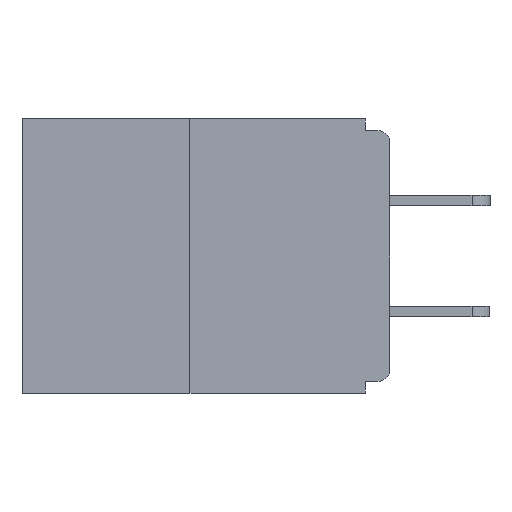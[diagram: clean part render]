
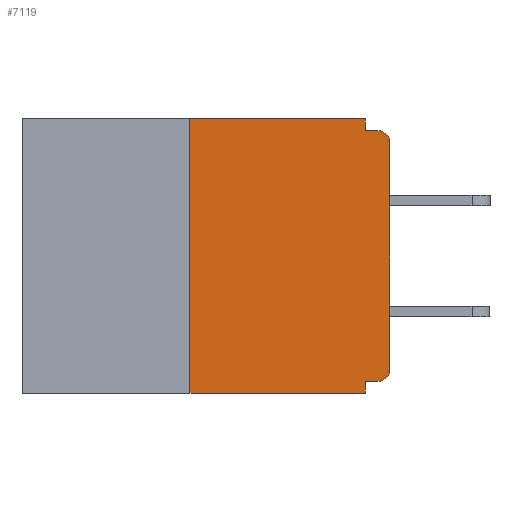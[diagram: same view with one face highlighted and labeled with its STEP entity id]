
A CAD part, left-side view. The second image highlights one B-rep face of the part: STEP entity #7119.
In plain terms, the highlighted planar face has unit normal (-1, 0, 0).
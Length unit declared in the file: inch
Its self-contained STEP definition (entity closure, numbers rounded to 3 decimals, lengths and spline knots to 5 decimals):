
#192 = DIRECTION ( 'NONE',  ( 0., 0., -1. ) ) ;
#366 = VECTOR ( 'NONE', #7528, 39.37008 ) ;
#459 = DIRECTION ( 'NONE',  ( 0., -1., 0. ) ) ;
#569 = LINE ( 'NONE', #3415, #7315 ) ;
#801 = DIRECTION ( 'NONE',  ( 0., 1., 0. ) ) ;
#1055 = LINE ( 'NONE', #1963, #10873 ) ;
#1112 = ORIENTED_EDGE ( 'NONE', *, *, #2928, .F. ) ;
#1185 = DIRECTION ( 'NONE',  ( 1., 0., 0. ) ) ;
#1282 = VERTEX_POINT ( 'NONE', #8384 ) ;
#1338 = CARTESIAN_POINT ( 'NONE',  ( 0., 0., -0.015 ) ) ;
#1354 = VERTEX_POINT ( 'NONE', #3255 ) ;
#1509 = EDGE_CURVE ( 'NONE', #8671, #5202, #1055, .T. ) ;
#1673 = EDGE_CURVE ( 'NONE', #11274, #4141, #1738, .T. ) ;
#1738 = LINE ( 'NONE', #6239, #3037 ) ;
#1742 = EDGE_CURVE ( 'NONE', #6405, #9979, #2314, .T. ) ;
#1790 = ORIENTED_EDGE ( 'NONE', *, *, #3524, .F. ) ;
#1808 = ORIENTED_EDGE ( 'NONE', *, *, #3674, .T. ) ;
#1810 = AXIS2_PLACEMENT_3D ( 'NONE', #3173, #2297, #4016 ) ;
#1963 = CARTESIAN_POINT ( 'NONE',  ( 0., 0.031, 0. ) ) ;
#2057 = ORIENTED_EDGE ( 'NONE', *, *, #8180, .T. ) ;
#2297 = DIRECTION ( 'NONE',  ( -1., 0., 0. ) ) ;
#2314 = LINE ( 'NONE', #3725, #11901 ) ;
#2386 = CARTESIAN_POINT ( 'NONE',  ( 0., 0.015, -0.03 ) ) ;
#2722 = EDGE_CURVE ( 'NONE', #5202, #1282, #6900, .T. ) ;
#2928 = EDGE_CURVE ( 'NONE', #4141, #7059, #10402, .T. ) ;
#3037 = VECTOR ( 'NONE', #801, 39.37008 ) ;
#3173 = CARTESIAN_POINT ( 'NONE',  ( 0., 0.015, -0.313 ) ) ;
#3252 = VECTOR ( 'NONE', #4634, 39.37008 ) ;
#3255 = CARTESIAN_POINT ( 'NONE',  ( 0., 0., -0.313 ) ) ;
#3415 = CARTESIAN_POINT ( 'NONE',  ( 0., 0.46, 0. ) ) ;
#3524 = EDGE_CURVE ( 'NONE', #9979, #8671, #569, .T. ) ;
#3625 = CARTESIAN_POINT ( 'NONE',  ( 0., 0., 0. ) ) ;
#3674 = EDGE_CURVE ( 'NONE', #1354, #5825, #11113, .T. ) ;
#3718 = CARTESIAN_POINT ( 'NONE',  ( 0., 0.46, 0. ) ) ;
#3725 = CARTESIAN_POINT ( 'NONE',  ( 0., 0.25, 0. ) ) ;
#3804 = CARTESIAN_POINT ( 'NONE',  ( 0., 0.25, 0. ) ) ;
#3908 = LINE ( 'NONE', #10203, #366 ) ;
#4016 = DIRECTION ( 'NONE',  ( 0., 0., -1. ) ) ;
#4094 = ORIENTED_EDGE ( 'NONE', *, *, #11140, .T. ) ;
#4135 = VECTOR ( 'NONE', #9179, 39.37008 ) ;
#4141 = VERTEX_POINT ( 'NONE', #4711 ) ;
#4213 = AXIS2_PLACEMENT_3D ( 'NONE', #2386, #11608, #8831 ) ;
#4394 = CARTESIAN_POINT ( 'NONE',  ( 0., 0.031, -0.343 ) ) ;
#4439 = VECTOR ( 'NONE', #459, 39.37008 ) ;
#4518 = DIRECTION ( 'NONE',  ( 0., 0., 1. ) ) ;
#4634 = DIRECTION ( 'NONE',  ( 0., 0., 1. ) ) ;
#4711 = CARTESIAN_POINT ( 'NONE',  ( 0., 0.031, -0.328 ) ) ;
#4747 = DIRECTION ( 'NONE',  ( 0., 0., -1. ) ) ;
#4833 = CARTESIAN_POINT ( 'NONE',  ( 0., 0.031, -0.015 ) ) ;
#4993 = CARTESIAN_POINT ( 'NONE',  ( 0., 0.031, 0. ) ) ;
#5202 = VERTEX_POINT ( 'NONE', #4833 ) ;
#5344 = DIRECTION ( 'NONE',  ( 0., -1., 0. ) ) ;
#5825 = VERTEX_POINT ( 'NONE', #10371 ) ;
#6092 = ORIENTED_EDGE ( 'NONE', *, *, #2722, .F. ) ;
#6239 = CARTESIAN_POINT ( 'NONE',  ( 0., 0., -0.328 ) ) ;
#6250 = CARTESIAN_POINT ( 'NONE',  ( 0., 0.015, -0.328 ) ) ;
#6405 = VERTEX_POINT ( 'NONE', #9694 ) ;
#6409 = ORIENTED_EDGE ( 'NONE', *, *, #6709, .T. ) ;
#6709 = EDGE_CURVE ( 'NONE', #6405, #7059, #3908, .T. ) ;
#6900 = LINE ( 'NONE', #1338, #4439 ) ;
#6943 = ORIENTED_EDGE ( 'NONE', *, *, #1742, .F. ) ;
#7059 = VERTEX_POINT ( 'NONE', #8942 ) ;
#7119 = ADVANCED_FACE ( 'NONE', ( #11750 ), #10239, .F. ) ;
#7315 = VECTOR ( 'NONE', #5344, 39.37008 ) ;
#7443 = ORIENTED_EDGE ( 'NONE', *, *, #1673, .F. ) ;
#7528 = DIRECTION ( 'NONE',  ( 0., -1., 0. ) ) ;
#8180 = EDGE_CURVE ( 'NONE', #11274, #1354, #10976, .T. ) ;
#8384 = CARTESIAN_POINT ( 'NONE',  ( 0., 0.015, -0.015 ) ) ;
#8436 = AXIS2_PLACEMENT_3D ( 'NONE', #3718, #1185, #192 ) ;
#8671 = VERTEX_POINT ( 'NONE', #4993 ) ;
#8831 = DIRECTION ( 'NONE',  ( 0., 0., -1. ) ) ;
#8913 = ORIENTED_EDGE ( 'NONE', *, *, #1509, .F. ) ;
#8942 = CARTESIAN_POINT ( 'NONE',  ( 0., 0.031, -0.343 ) ) ;
#9179 = DIRECTION ( 'NONE',  ( 0., 0., -1. ) ) ;
#9694 = CARTESIAN_POINT ( 'NONE',  ( 0., 0.25, -0.343 ) ) ;
#9979 = VERTEX_POINT ( 'NONE', #3804 ) ;
#10203 = CARTESIAN_POINT ( 'NONE',  ( 0., 0.46, -0.343 ) ) ;
#10239 = PLANE ( 'NONE',  #8436 ) ;
#10348 = CIRCLE ( 'NONE', #4213, 0.015 ) ;
#10371 = CARTESIAN_POINT ( 'NONE',  ( 0., 0., -0.03 ) ) ;
#10402 = LINE ( 'NONE', #4394, #4135 ) ;
#10536 = EDGE_LOOP ( 'NONE', ( #1790, #6943, #6409, #1112, #7443, #2057, #1808, #4094, #6092, #8913 ) ) ;
#10873 = VECTOR ( 'NONE', #4747, 39.37008 ) ;
#10976 = CIRCLE ( 'NONE', #1810, 0.015 ) ;
#11113 = LINE ( 'NONE', #3625, #3252 ) ;
#11140 = EDGE_CURVE ( 'NONE', #5825, #1282, #10348, .T. ) ;
#11274 = VERTEX_POINT ( 'NONE', #6250 ) ;
#11608 = DIRECTION ( 'NONE',  ( -1., 0., 0. ) ) ;
#11750 = FACE_OUTER_BOUND ( 'NONE', #10536, .T. ) ;
#11901 = VECTOR ( 'NONE', #4518, 39.37008 ) ;
